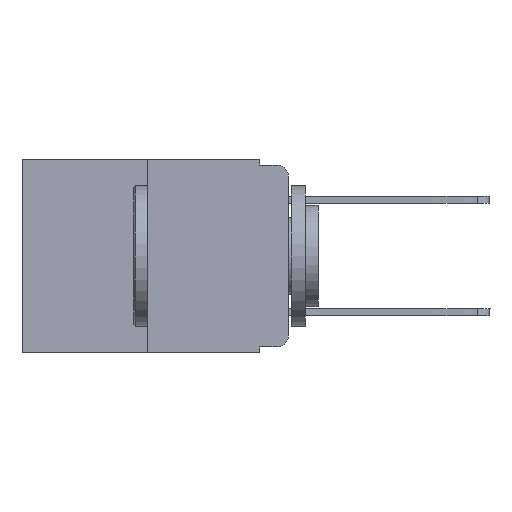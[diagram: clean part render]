
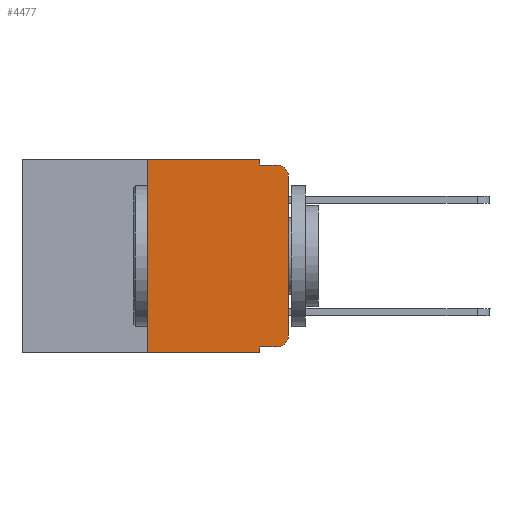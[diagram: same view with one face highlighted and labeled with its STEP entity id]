
A CAD part, left-side view. The second image highlights one B-rep face of the part: STEP entity #4477.
In plain terms, the highlighted planar face has unit normal (-1, 0, 0).
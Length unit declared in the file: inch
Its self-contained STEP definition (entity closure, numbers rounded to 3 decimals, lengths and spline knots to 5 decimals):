
#140 = VERTEX_POINT ( 'NONE', #9771 ) ;
#315 = CIRCLE ( 'NONE', #20862, 0.02 ) ;
#497 = LINE ( 'NONE', #1701, #15125 ) ;
#726 = DIRECTION ( 'NONE',  ( 0., 0., -1. ) ) ;
#1322 = EDGE_CURVE ( 'NONE', #4062, #13505, #315, .T. ) ;
#1326 = ORIENTED_EDGE ( 'NONE', *, *, #8712, .F. ) ;
#1574 = VECTOR ( 'NONE', #13525, 39.37008 ) ;
#1701 = CARTESIAN_POINT ( 'NONE',  ( 0., 0.473, 0. ) ) ;
#1885 = DIRECTION ( 'NONE',  ( 0., 0., 1. ) ) ;
#2128 = ORIENTED_EDGE ( 'NONE', *, *, #20945, .F. ) ;
#2909 = VECTOR ( 'NONE', #1885, 39.37008 ) ;
#2921 = VECTOR ( 'NONE', #10452, 39.37008 ) ;
#3072 = VERTEX_POINT ( 'NONE', #18224 ) ;
#3301 = LINE ( 'NONE', #10160, #2909 ) ;
#3461 = CARTESIAN_POINT ( 'NONE',  ( 0., 0.473, -0.343 ) ) ;
#3561 = LINE ( 'NONE', #3461, #19283 ) ;
#3746 = LINE ( 'NONE', #20204, #9828 ) ;
#3761 = CARTESIAN_POINT ( 'NONE',  ( 0., 0.25, -0.343 ) ) ;
#4062 = VERTEX_POINT ( 'NONE', #13908 ) ;
#4098 = CARTESIAN_POINT ( 'NONE',  ( 0., 0.02, -0.03 ) ) ;
#4162 = CARTESIAN_POINT ( 'NONE',  ( 0., 0.051, 0. ) ) ;
#4477 = ADVANCED_FACE ( 'NONE', ( #7327 ), #20642, .F. ) ;
#5700 = CARTESIAN_POINT ( 'NONE',  ( 0., 0.473, 0. ) ) ;
#5802 = DIRECTION ( 'NONE',  ( 0., 0., -1. ) ) ;
#6270 = DIRECTION ( 'NONE',  ( 0., 0., -1. ) ) ;
#6909 = DIRECTION ( 'NONE',  ( 0., -1., 0. ) ) ;
#6940 = DIRECTION ( 'NONE',  ( 0., -1., 0. ) ) ;
#7327 = FACE_OUTER_BOUND ( 'NONE', #19499, .T. ) ;
#7451 = CIRCLE ( 'NONE', #19652, 0.02 ) ;
#7492 = VECTOR ( 'NONE', #9076, 39.37008 ) ;
#8468 = ORIENTED_EDGE ( 'NONE', *, *, #21143, .F. ) ;
#8712 = EDGE_CURVE ( 'NONE', #12723, #3072, #14281, .T. ) ;
#8941 = CARTESIAN_POINT ( 'NONE',  ( 0., 0.02, -0.01 ) ) ;
#9076 = DIRECTION ( 'NONE',  ( 0., 0., -1. ) ) ;
#9378 = VERTEX_POINT ( 'NONE', #16841 ) ;
#9676 = AXIS2_PLACEMENT_3D ( 'NONE', #5700, #10726, #17340 ) ;
#9771 = CARTESIAN_POINT ( 'NONE',  ( 0., 0.25, 0. ) ) ;
#9828 = VECTOR ( 'NONE', #9957, 39.37008 ) ;
#9957 = DIRECTION ( 'NONE',  ( 0., -1., 0. ) ) ;
#10010 = CARTESIAN_POINT ( 'NONE',  ( 0., 0., 0. ) ) ;
#10160 = CARTESIAN_POINT ( 'NONE',  ( 0., 0.25, 0. ) ) ;
#10452 = DIRECTION ( 'NONE',  ( 0., 0., 1. ) ) ;
#10660 = ORIENTED_EDGE ( 'NONE', *, *, #1322, .T. ) ;
#10726 = DIRECTION ( 'NONE',  ( 1., 0., 0. ) ) ;
#10741 = ORIENTED_EDGE ( 'NONE', *, *, #15106, .T. ) ;
#10743 = DIRECTION ( 'NONE',  ( -1., 0., 0. ) ) ;
#11313 = ORIENTED_EDGE ( 'NONE', *, *, #12582, .T. ) ;
#12445 = LINE ( 'NONE', #4162, #7492 ) ;
#12582 = EDGE_CURVE ( 'NONE', #19931, #9378, #3746, .T. ) ;
#12723 = VERTEX_POINT ( 'NONE', #20856 ) ;
#13505 = VERTEX_POINT ( 'NONE', #8941 ) ;
#13525 = DIRECTION ( 'NONE',  ( 0., -1., 0. ) ) ;
#13634 = CARTESIAN_POINT ( 'NONE',  ( 0., 0.051, -0.01 ) ) ;
#13908 = CARTESIAN_POINT ( 'NONE',  ( 0., 0., -0.03 ) ) ;
#14281 = LINE ( 'NONE', #20747, #14690 ) ;
#14686 = EDGE_CURVE ( 'NONE', #19312, #140, #3301, .T. ) ;
#14690 = VECTOR ( 'NONE', #5802, 39.37008 ) ;
#14946 = LINE ( 'NONE', #13634, #1574 ) ;
#15106 = EDGE_CURVE ( 'NONE', #19312, #19504, #3561, .T. ) ;
#15111 = EDGE_CURVE ( 'NONE', #17569, #4062, #18272, .T. ) ;
#15125 = VECTOR ( 'NONE', #6909, 39.37008 ) ;
#15926 = ORIENTED_EDGE ( 'NONE', *, *, #20352, .T. ) ;
#16841 = CARTESIAN_POINT ( 'NONE',  ( 0., 0.02, -0.333 ) ) ;
#17340 = DIRECTION ( 'NONE',  ( 0., 0., -1. ) ) ;
#17569 = VERTEX_POINT ( 'NONE', #20044 ) ;
#17598 = ORIENTED_EDGE ( 'NONE', *, *, #15111, .T. ) ;
#18139 = ORIENTED_EDGE ( 'NONE', *, *, #14686, .F. ) ;
#18224 = CARTESIAN_POINT ( 'NONE',  ( 0., 0.051, -0.01 ) ) ;
#18272 = LINE ( 'NONE', #10010, #2921 ) ;
#19283 = VECTOR ( 'NONE', #6940, 39.37008 ) ;
#19312 = VERTEX_POINT ( 'NONE', #3761 ) ;
#19499 = EDGE_LOOP ( 'NONE', ( #17598, #10660, #2128, #1326, #21484, #18139, #10741, #8468, #11313, #15926 ) ) ;
#19504 = VERTEX_POINT ( 'NONE', #21399 ) ;
#19652 = AXIS2_PLACEMENT_3D ( 'NONE', #21540, #21221, #6270 ) ;
#19931 = VERTEX_POINT ( 'NONE', #20939 ) ;
#20044 = CARTESIAN_POINT ( 'NONE',  ( 0., 0., -0.313 ) ) ;
#20204 = CARTESIAN_POINT ( 'NONE',  ( 0., 0.051, -0.333 ) ) ;
#20352 = EDGE_CURVE ( 'NONE', #9378, #17569, #7451, .T. ) ;
#20589 = EDGE_CURVE ( 'NONE', #140, #12723, #497, .T. ) ;
#20642 = PLANE ( 'NONE',  #9676 ) ;
#20747 = CARTESIAN_POINT ( 'NONE',  ( 0., 0.051, 0. ) ) ;
#20856 = CARTESIAN_POINT ( 'NONE',  ( 0., 0.051, 0. ) ) ;
#20862 = AXIS2_PLACEMENT_3D ( 'NONE', #4098, #10743, #726 ) ;
#20939 = CARTESIAN_POINT ( 'NONE',  ( 0., 0.051, -0.333 ) ) ;
#20945 = EDGE_CURVE ( 'NONE', #3072, #13505, #14946, .T. ) ;
#21143 = EDGE_CURVE ( 'NONE', #19931, #19504, #12445, .T. ) ;
#21221 = DIRECTION ( 'NONE',  ( -1., 0., 0. ) ) ;
#21399 = CARTESIAN_POINT ( 'NONE',  ( 0., 0.051, -0.343 ) ) ;
#21484 = ORIENTED_EDGE ( 'NONE', *, *, #20589, .F. ) ;
#21540 = CARTESIAN_POINT ( 'NONE',  ( 0., 0.02, -0.313 ) ) ;
